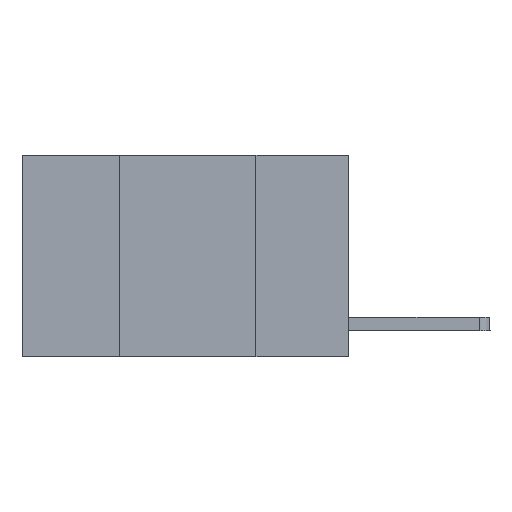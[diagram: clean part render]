
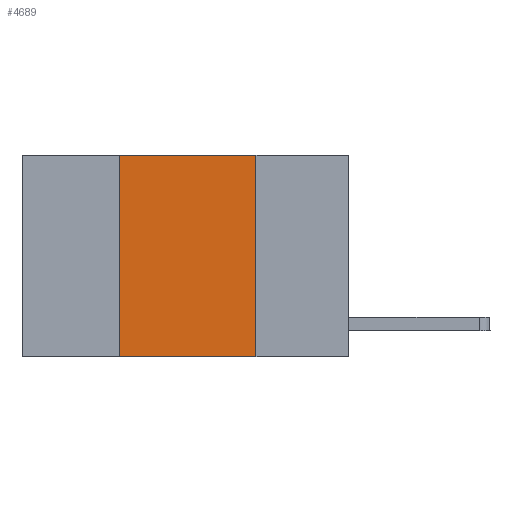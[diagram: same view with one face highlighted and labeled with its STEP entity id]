
A CAD part, left-side view. The second image highlights one B-rep face of the part: STEP entity #4689.
In plain terms, the highlighted planar face has unit normal (-1, 0, 0).
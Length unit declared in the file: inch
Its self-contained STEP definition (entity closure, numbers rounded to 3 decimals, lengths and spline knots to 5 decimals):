
#486 = ORIENTED_EDGE ( 'NONE', *, *, #7928, .T. ) ;
#1152 = CARTESIAN_POINT ( 'NONE',  ( 0., 0.42, -0.37 ) ) ;
#1438 = FACE_OUTER_BOUND ( 'NONE', #6949, .T. ) ;
#1641 = VECTOR ( 'NONE', #7446, 39.37008 ) ;
#1648 = LINE ( 'NONE', #7545, #1641 ) ;
#1759 = VERTEX_POINT ( 'NONE', #5848 ) ;
#2078 = ORIENTED_EDGE ( 'NONE', *, *, #5257, .F. ) ;
#2210 = EDGE_CURVE ( 'NONE', #4114, #1759, #8816, .T. ) ;
#2394 = LINE ( 'NONE', #8271, #5775 ) ;
#2491 = EDGE_CURVE ( 'NONE', #2706, #6970, #3668, .T. ) ;
#2706 = VERTEX_POINT ( 'NONE', #1152 ) ;
#3668 = LINE ( 'NONE', #4426, #9320 ) ;
#3971 = ORIENTED_EDGE ( 'NONE', *, *, #2210, .F. ) ;
#4049 = CARTESIAN_POINT ( 'NONE',  ( 0., 0.17, 0. ) ) ;
#4114 = VERTEX_POINT ( 'NONE', #4049 ) ;
#4426 = CARTESIAN_POINT ( 'NONE',  ( 0., 0.42, 0. ) ) ;
#4689 = ADVANCED_FACE ( 'NONE', ( #1438 ), #8144, .F. ) ;
#5257 = EDGE_CURVE ( 'NONE', #6970, #4114, #1648, .T. ) ;
#5636 = AXIS2_PLACEMENT_3D ( 'NONE', #6597, #8049, #5831 ) ;
#5727 = ORIENTED_EDGE ( 'NONE', *, *, #2491, .F. ) ;
#5775 = VECTOR ( 'NONE', #8130, 39.37008 ) ;
#5831 = DIRECTION ( 'NONE',  ( 0., 0., -1. ) ) ;
#5848 = CARTESIAN_POINT ( 'NONE',  ( 0., 0.17, -0.37 ) ) ;
#6597 = CARTESIAN_POINT ( 'NONE',  ( 0., 0.6, 0. ) ) ;
#6610 = CARTESIAN_POINT ( 'NONE',  ( 0., 0.42, 0. ) ) ;
#6949 = EDGE_LOOP ( 'NONE', ( #3971, #2078, #5727, #486 ) ) ;
#6970 = VERTEX_POINT ( 'NONE', #6610 ) ;
#7282 = DIRECTION ( 'NONE',  ( 0., 0., -1. ) ) ;
#7315 = VECTOR ( 'NONE', #7282, 39.37008 ) ;
#7446 = DIRECTION ( 'NONE',  ( 0., -1., 0. ) ) ;
#7545 = CARTESIAN_POINT ( 'NONE',  ( 0., 0.6, 0. ) ) ;
#7928 = EDGE_CURVE ( 'NONE', #2706, #1759, #2394, .T. ) ;
#8049 = DIRECTION ( 'NONE',  ( 1., 0., 0. ) ) ;
#8130 = DIRECTION ( 'NONE',  ( 0., -1., 0. ) ) ;
#8144 = PLANE ( 'NONE',  #5636 ) ;
#8154 = CARTESIAN_POINT ( 'NONE',  ( 0., 0.17, 0. ) ) ;
#8271 = CARTESIAN_POINT ( 'NONE',  ( 0., 0.6, -0.37 ) ) ;
#8704 = DIRECTION ( 'NONE',  ( 0., 0., 1. ) ) ;
#8816 = LINE ( 'NONE', #8154, #7315 ) ;
#9320 = VECTOR ( 'NONE', #8704, 39.37008 ) ;
